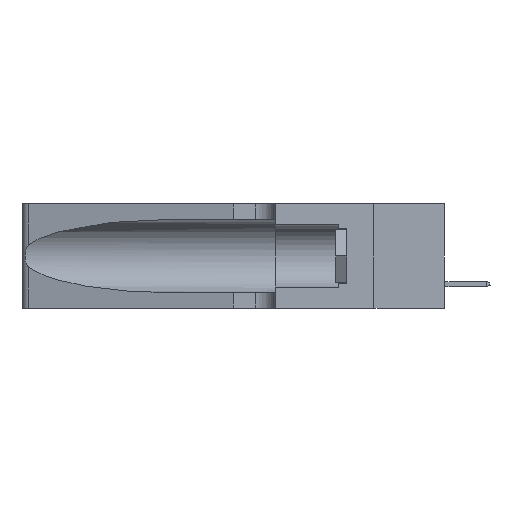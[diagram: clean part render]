
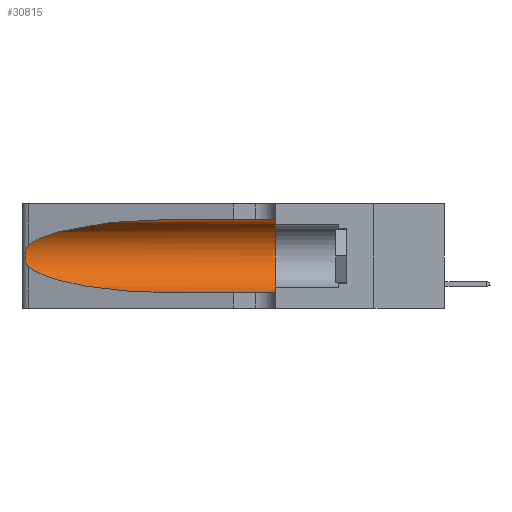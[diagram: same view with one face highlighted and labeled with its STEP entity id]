
A CAD part, left-side view. The second image highlights one B-rep face of the part: STEP entity #30815.
In plain terms, the highlighted cylindrical face has radius 3.308 mm (diameter 6.617 mm), a partial arc.
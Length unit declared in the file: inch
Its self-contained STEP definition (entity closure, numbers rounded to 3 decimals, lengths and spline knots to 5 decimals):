
#434 = CIRCLE ( 'NONE', #12401, 0.13025 ) ;
#468 = CARTESIAN_POINT ( 'NONE',  ( 0.1305, 1.61858, 0.185 ) ) ;
#597 = ORIENTED_EDGE ( 'NONE', *, *, #25787, .T. ) ;
#1909 = CARTESIAN_POINT ( 'NONE',  ( 0.25854, 1.2359, 0.20912 ) ) ;
#2090 = CARTESIAN_POINT ( 'NONE',  ( 0.25639, 1.23184, 0.21858 ) ) ;
#2132 = VERTEX_POINT ( 'NONE', #29936 ) ;
#2249 = DIRECTION ( 'NONE',  ( 0., -1., 0. ) ) ;
#3104 = CARTESIAN_POINT ( 'NONE',  ( 0.25639, 1.23186, 0.15144 ) ) ;
#4533 = VERTEX_POINT ( 'NONE', #34191 ) ;
#4542 = EDGE_CURVE ( 'NONE', #18476, #2132, #28144, .T. ) ;
#5823 = CARTESIAN_POINT ( 'NONE',  ( 0.26075, 1.23896, 0.19203 ) ) ;
#7147 = CARTESIAN_POINT ( 'NONE',  ( 0.25487, 1.22718, 0.14631 ) ) ;
#7640 = ORIENTED_EDGE ( 'NONE', *, *, #8308, .F. ) ;
#8308 = EDGE_CURVE ( 'NONE', #49243, #4533, #14862, .T. ) ;
#9684 = CARTESIAN_POINT ( 'NONE',  ( 0.1305, 1.61858, 0.05475 ) ) ;
#9877 = CARTESIAN_POINT ( 'NONE',  ( 0.25487, 1.22718, 0.22369 ) ) ;
#11795 = ORIENTED_EDGE ( 'NONE', *, *, #40627, .T. ) ;
#11939 = DIRECTION ( 'NONE',  ( 0., -1., 0. ) ) ;
#12401 = AXIS2_PLACEMENT_3D ( 'NONE', #49224, #18255, #25879 ) ;
#12831 = ORIENTED_EDGE ( 'NONE', *, *, #30506, .F. ) ;
#13051 = VERTEX_POINT ( 'NONE', #48329 ) ;
#13845 = CARTESIAN_POINT ( 'NONE',  ( 0.25487, 1.22718, 0.22369 ) ) ;
#14862 = LINE ( 'NONE', #31043, #30140 ) ;
#16015 = DIRECTION ( 'NONE',  ( 0., -1., 0. ) ) ;
#17919 = ORIENTED_EDGE ( 'NONE', *, *, #33066, .T. ) ;
#18213 = VERTEX_POINT ( 'NONE', #13845 ) ;
#18255 = DIRECTION ( 'NONE',  ( 0., 1., 0. ) ) ;
#18476 = VERTEX_POINT ( 'NONE', #7147 ) ;
#19123 = AXIS2_PLACEMENT_3D ( 'NONE', #468, #16015, #43240 ) ;
#19639 = CARTESIAN_POINT ( 'NONE',  ( 0.1305, 0.72297, 0.31525 ) ) ;
#19904 = EDGE_LOOP ( 'NONE', ( #11795, #597, #48062, #17919, #12831, #7640 ) ) ;
#21015 = VECTOR ( 'NONE', #2249, 39.37008 ) ;
#22039 = CARTESIAN_POINT ( 'NONE',  ( 0.25487, 1.22718, 0.14631 ) ) ;
#22732 = CARTESIAN_POINT ( 'NONE',  ( 0.25856, 1.23593, 0.16098 ) ) ;
#23739 =( BOUNDED_CURVE ( )  B_SPLINE_CURVE ( 3, ( #19639, #39209, #42785, #43273 ),
 .UNSPECIFIED., .F., .F. ) 
 B_SPLINE_CURVE_WITH_KNOTS ( ( 4, 4 ),
 ( 1.5708, 2.84003 ),
 .UNSPECIFIED. ) 
 CURVE ( )  GEOMETRIC_REPRESENTATION_ITEM ( )  RATIONAL_B_SPLINE_CURVE ( ( 1., 0.87, 0.87, 1. ) ) 
 REPRESENTATION_ITEM ( '' )  );
#24573 = CARTESIAN_POINT ( 'NONE',  ( 0.1305, 0.72297, 0.31525 ) ) ;
#25250 = CARTESIAN_POINT ( 'NONE',  ( 0.25787, 1.23484, 0.2124 ) ) ;
#25409 = CARTESIAN_POINT ( 'NONE',  ( 0.25555, 1.22994, 0.2215 ) ) ;
#25787 = EDGE_CURVE ( 'NONE', #18213, #18476, #39376, .T. ) ;
#25879 = DIRECTION ( 'NONE',  ( 0., 0., 1. ) ) ;
#26438 = CARTESIAN_POINT ( 'NONE',  ( 0.26017, 1.23833, 0.17102 ) ) ;
#26715 = CYLINDRICAL_SURFACE ( 'NONE', #19123, 0.13025 ) ;
#28144 =( BOUNDED_CURVE ( )  B_SPLINE_CURVE ( 3, ( #34353, #50027, #30649, #42377 ),
 .UNSPECIFIED., .F., .F. ) 
 B_SPLINE_CURVE_WITH_KNOTS ( ( 4, 4 ),
 ( 3.44316, 4.71239 ),
 .UNSPECIFIED. ) 
 CURVE ( )  GEOMETRIC_REPRESENTATION_ITEM ( )  RATIONAL_B_SPLINE_CURVE ( ( 1., 0.87, 0.87, 1. ) ) 
 REPRESENTATION_ITEM ( '' )  );
#29208 = CARTESIAN_POINT ( 'NONE',  ( 0.26018, 1.23835, 0.19895 ) ) ;
#29936 = CARTESIAN_POINT ( 'NONE',  ( 0.1305, 0.72297, 0.05475 ) ) ;
#30140 = VECTOR ( 'NONE', #11939, 39.37008 ) ;
#30396 = CARTESIAN_POINT ( 'NONE',  ( 0.25555, 1.22993, 0.14849 ) ) ;
#30506 = EDGE_CURVE ( 'NONE', #4533, #13051, #434, .T. ) ;
#30649 = CARTESIAN_POINT ( 'NONE',  ( 0.18966, 0.96281, 0.05475 ) ) ;
#30815 = ADVANCED_FACE ( 'NONE', ( #43713 ), #26715, .F. ) ;
#31043 = CARTESIAN_POINT ( 'NONE',  ( 0.1305, 1.61858, 0.31525 ) ) ;
#33066 = EDGE_CURVE ( 'NONE', #2132, #13051, #38068, .T. ) ;
#33930 = CARTESIAN_POINT ( 'NONE',  ( 0.25789, 1.23486, 0.15765 ) ) ;
#34191 = CARTESIAN_POINT ( 'NONE',  ( 0.1305, 0.35, 0.31525 ) ) ;
#34353 = CARTESIAN_POINT ( 'NONE',  ( 0.25487, 1.22718, 0.14631 ) ) ;
#38068 = LINE ( 'NONE', #9684, #21015 ) ;
#39209 = CARTESIAN_POINT ( 'NONE',  ( 0.18966, 0.96281, 0.31525 ) ) ;
#39376 = B_SPLINE_CURVE_WITH_KNOTS ( 'NONE', 3,
 ( #9877, #25409, #2090, #25250, #1909, #29208, #5823, #49775, #26438, #22732, #33930, #3104, #30396, #22039 ),
 .UNSPECIFIED., .F., .F.,
 ( 4, 2, 2, 2, 2, 2, 4 ),
 ( 0., 0.00027, 0.00053, 0.00107, 0.0016, 0.00187, 0.00214 ),
 .UNSPECIFIED. ) ;
#40627 = EDGE_CURVE ( 'NONE', #49243, #18213, #23739, .T. ) ;
#42377 = CARTESIAN_POINT ( 'NONE',  ( 0.1305, 0.72297, 0.05475 ) ) ;
#42785 = CARTESIAN_POINT ( 'NONE',  ( 0.2373, 1.15595, 0.28018 ) ) ;
#43240 = DIRECTION ( 'NONE',  ( 0., 0., -1. ) ) ;
#43273 = CARTESIAN_POINT ( 'NONE',  ( 0.25487, 1.22718, 0.22369 ) ) ;
#43713 = FACE_OUTER_BOUND ( 'NONE', #19904, .T. ) ;
#48062 = ORIENTED_EDGE ( 'NONE', *, *, #4542, .T. ) ;
#48329 = CARTESIAN_POINT ( 'NONE',  ( 0.1305, 0.35, 0.05475 ) ) ;
#49224 = CARTESIAN_POINT ( 'NONE',  ( 0.1305, 0.35, 0.185 ) ) ;
#49243 = VERTEX_POINT ( 'NONE', #24573 ) ;
#49775 = CARTESIAN_POINT ( 'NONE',  ( 0.26075, 1.23896, 0.178 ) ) ;
#50027 = CARTESIAN_POINT ( 'NONE',  ( 0.2373, 1.15595, 0.08982 ) ) ;
